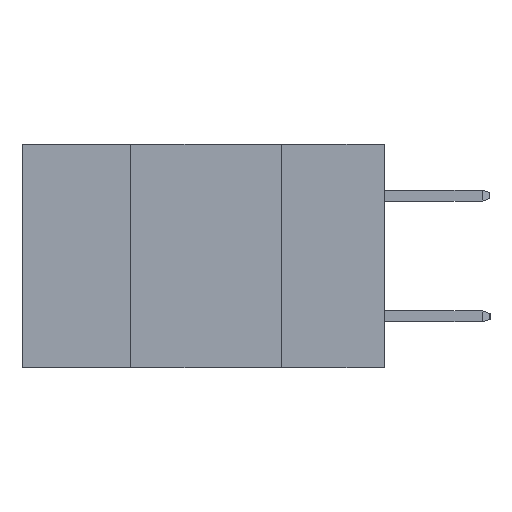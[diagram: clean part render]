
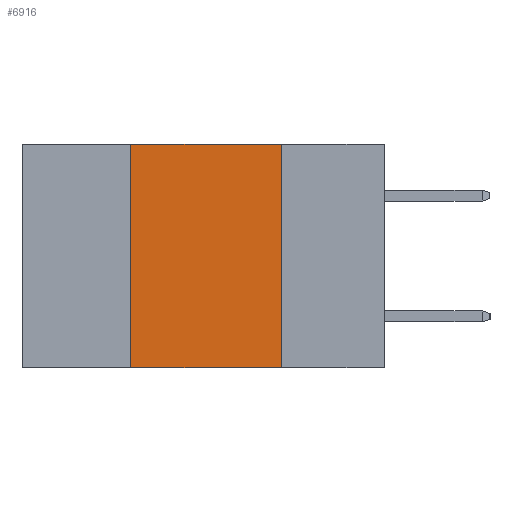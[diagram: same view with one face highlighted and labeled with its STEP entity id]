
A CAD part, left-side view. The second image highlights one B-rep face of the part: STEP entity #6916.
In plain terms, the highlighted planar face has unit normal (-1, 0, 0).
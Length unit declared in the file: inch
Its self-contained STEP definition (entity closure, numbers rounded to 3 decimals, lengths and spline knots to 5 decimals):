
#75 = CARTESIAN_POINT ( 'NONE',  ( 0., 0.6, 0. ) ) ;
#122 = EDGE_CURVE ( 'NONE', #7352, #6003, #8036, .T. ) ;
#195 = PLANE ( 'NONE',  #6264 ) ;
#1923 = EDGE_CURVE ( 'NONE', #8845, #7080, #10329, .T. ) ;
#2154 = CARTESIAN_POINT ( 'NONE',  ( 0., 0.6, 0. ) ) ;
#2170 = DIRECTION ( 'NONE',  ( 0., -1., 0. ) ) ;
#2580 = ORIENTED_EDGE ( 'NONE', *, *, #9966, .F. ) ;
#3587 = ORIENTED_EDGE ( 'NONE', *, *, #13311, .T. ) ;
#3935 = CARTESIAN_POINT ( 'NONE',  ( 0., 0.6, -0.37 ) ) ;
#4100 = DIRECTION ( 'NONE',  ( 0., -1., 0. ) ) ;
#4735 = LINE ( 'NONE', #3935, #10655 ) ;
#5482 = ORIENTED_EDGE ( 'NONE', *, *, #122, .F. ) ;
#5718 = CARTESIAN_POINT ( 'NONE',  ( 0., 0.17, -0.37 ) ) ;
#5994 = DIRECTION ( 'NONE',  ( 0., 0., 1. ) ) ;
#6003 = VERTEX_POINT ( 'NONE', #5718 ) ;
#6009 = CARTESIAN_POINT ( 'NONE',  ( 0., 0.42, -0.37 ) ) ;
#6067 = ORIENTED_EDGE ( 'NONE', *, *, #1923, .F. ) ;
#6264 = AXIS2_PLACEMENT_3D ( 'NONE', #75, #15024, #15012 ) ;
#6916 = ADVANCED_FACE ( 'NONE', ( #9437 ), #195, .F. ) ;
#7080 = VERTEX_POINT ( 'NONE', #12534 ) ;
#7352 = VERTEX_POINT ( 'NONE', #8604 ) ;
#7708 = CARTESIAN_POINT ( 'NONE',  ( 0., 0.17, -0.37 ) ) ;
#8036 = LINE ( 'NONE', #7708, #13762 ) ;
#8604 = CARTESIAN_POINT ( 'NONE',  ( 0., 0.17, 0. ) ) ;
#8845 = VERTEX_POINT ( 'NONE', #11256 ) ;
#9437 = FACE_OUTER_BOUND ( 'NONE', #12394, .T. ) ;
#9480 = LINE ( 'NONE', #2154, #12870 ) ;
#9966 = EDGE_CURVE ( 'NONE', #7080, #7352, #9480, .T. ) ;
#9979 = VECTOR ( 'NONE', #5994, 39.37008 ) ;
#10329 = LINE ( 'NONE', #6009, #9979 ) ;
#10655 = VECTOR ( 'NONE', #4100, 39.37008 ) ;
#11256 = CARTESIAN_POINT ( 'NONE',  ( 0., 0.42, -0.37 ) ) ;
#11854 = DIRECTION ( 'NONE',  ( 0., 0., -1. ) ) ;
#12394 = EDGE_LOOP ( 'NONE', ( #5482, #2580, #6067, #3587 ) ) ;
#12534 = CARTESIAN_POINT ( 'NONE',  ( 0., 0.42, 0. ) ) ;
#12870 = VECTOR ( 'NONE', #2170, 39.37008 ) ;
#13311 = EDGE_CURVE ( 'NONE', #8845, #6003, #4735, .T. ) ;
#13762 = VECTOR ( 'NONE', #11854, 39.37008 ) ;
#15012 = DIRECTION ( 'NONE',  ( 0., 0., -1. ) ) ;
#15024 = DIRECTION ( 'NONE',  ( 1., 0., 0. ) ) ;
